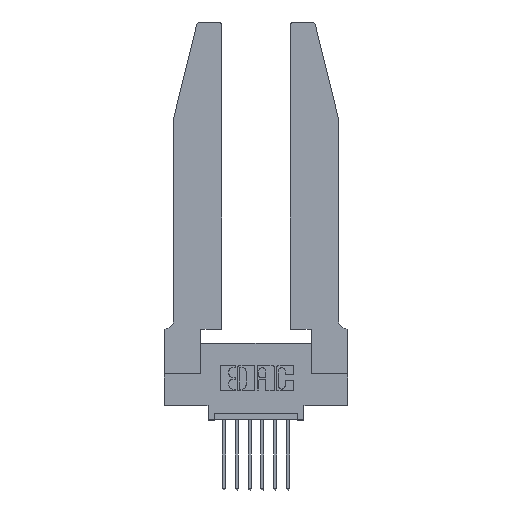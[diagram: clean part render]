
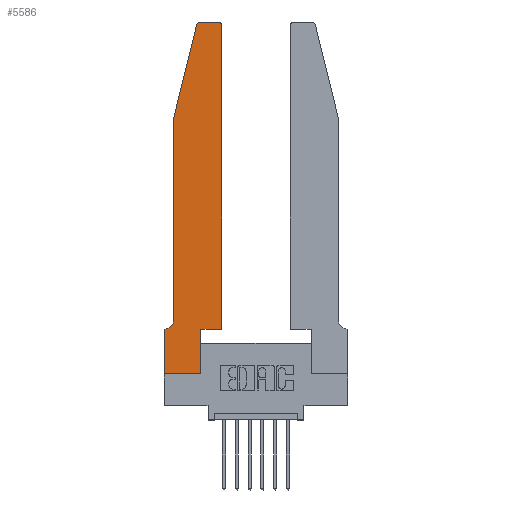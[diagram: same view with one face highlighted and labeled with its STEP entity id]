
A CAD part, top view. The second image highlights one B-rep face of the part: STEP entity #5586.
In plain terms, the highlighted planar face has unit normal (0, 0, 1).
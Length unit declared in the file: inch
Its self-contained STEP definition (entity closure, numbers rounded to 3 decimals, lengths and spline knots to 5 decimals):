
#193 = CARTESIAN_POINT ( 'NONE',  ( 0.4505, 2.72, 0.37 ) ) ;
#317 = EDGE_CURVE ( 'NONE', #8953, #6873, #13744, .T. ) ;
#585 = DIRECTION ( 'NONE',  ( 0., 1., 0. ) ) ;
#881 = CARTESIAN_POINT ( 'NONE',  ( 0.0055, 0.35, 0.37 ) ) ;
#1132 = DIRECTION ( 'NONE',  ( 1., 0., 0. ) ) ;
#1405 = VERTEX_POINT ( 'NONE', #6700 ) ;
#1771 = EDGE_CURVE ( 'NONE', #5127, #13614, #2562, .T. ) ;
#1801 = VECTOR ( 'NONE', #3980, 39.37008 ) ;
#2337 = DIRECTION ( 'NONE',  ( -1., 0., 0. ) ) ;
#2392 = CARTESIAN_POINT ( 'NONE',  ( 0.0755, 0.35, 0.37 ) ) ;
#2511 = LINE ( 'NONE', #11585, #11950 ) ;
#2553 = DIRECTION ( 'NONE',  ( 0., 1., 0. ) ) ;
#2562 = LINE ( 'NONE', #3612, #6663 ) ;
#2755 = VERTEX_POINT ( 'NONE', #8130 ) ;
#2925 = VECTOR ( 'NONE', #13827, 39.37008 ) ;
#3608 = EDGE_CURVE ( 'NONE', #11274, #7448, #2511, .T. ) ;
#3612 = CARTESIAN_POINT ( 'NONE',  ( 0., 0., 0.37 ) ) ;
#3656 = CARTESIAN_POINT ( 'NONE',  ( 0.0755, 2., 0.37 ) ) ;
#3699 = VECTOR ( 'NONE', #13794, 39.37008 ) ;
#3912 = CARTESIAN_POINT ( 'NONE',  ( 0., 0.35, 0.37 ) ) ;
#3980 = DIRECTION ( 'NONE',  ( 1., 0., 0. ) ) ;
#4232 = AXIS2_PLACEMENT_3D ( 'NONE', #11447, #13595, #7993 ) ;
#4263 = DIRECTION ( 'NONE',  ( 0., 0., 1. ) ) ;
#4504 = ORIENTED_EDGE ( 'NONE', *, *, #13105, .T. ) ;
#4543 = EDGE_CURVE ( 'NONE', #13614, #11274, #11065, .T. ) ;
#4575 = EDGE_CURVE ( 'NONE', #5020, #2755, #6593, .T. ) ;
#4583 = VECTOR ( 'NONE', #9772, 39.37008 ) ;
#4726 = EDGE_CURVE ( 'NONE', #6873, #5210, #8148, .T. ) ;
#4813 = LINE ( 'NONE', #9290, #2925 ) ;
#4885 = EDGE_CURVE ( 'NONE', #2755, #11107, #7281, .T. ) ;
#5020 = VERTEX_POINT ( 'NONE', #12413 ) ;
#5127 = VERTEX_POINT ( 'NONE', #3912 ) ;
#5210 = VERTEX_POINT ( 'NONE', #13983 ) ;
#5295 = VECTOR ( 'NONE', #2553, 39.37008 ) ;
#5488 = AXIS2_PLACEMENT_3D ( 'NONE', #7690, #4263, #1132 ) ;
#5586 = ADVANCED_FACE ( 'NONE', ( #7943 ), #8099, .T. ) ;
#5783 = CARTESIAN_POINT ( 'NONE',  ( 0., 0., 0.37 ) ) ;
#5892 = ORIENTED_EDGE ( 'NONE', *, *, #4575, .T. ) ;
#5915 = VERTEX_POINT ( 'NONE', #9154 ) ;
#6064 = CARTESIAN_POINT ( 'NONE',  ( 0.2865, 0.35, 0.37 ) ) ;
#6113 = DIRECTION ( 'NONE',  ( 0., 0., 1. ) ) ;
#6593 = LINE ( 'NONE', #8356, #3699 ) ;
#6663 = VECTOR ( 'NONE', #12492, 39.37008 ) ;
#6700 = CARTESIAN_POINT ( 'NONE',  ( 0.25487, 2.72718, 0.37 ) ) ;
#6873 = VERTEX_POINT ( 'NONE', #193 ) ;
#6919 = CARTESIAN_POINT ( 'NONE',  ( 0.4505, 0.35, 0.37 ) ) ;
#7006 = CARTESIAN_POINT ( 'NONE',  ( 0., 0., 0.37 ) ) ;
#7033 = EDGE_CURVE ( 'NONE', #7448, #8953, #4813, .T. ) ;
#7281 = CIRCLE ( 'NONE', #14024, 0.07 ) ;
#7448 = VERTEX_POINT ( 'NONE', #6064 ) ;
#7690 = CARTESIAN_POINT ( 'NONE',  ( 0.4205, 2.72, 0.37 ) ) ;
#7939 = DIRECTION ( 'NONE',  ( 0., 0., -1. ) ) ;
#7943 = FACE_OUTER_BOUND ( 'NONE', #8574, .T. ) ;
#7993 = DIRECTION ( 'NONE',  ( 1., 0., 0. ) ) ;
#8099 = PLANE ( 'NONE',  #4232 ) ;
#8130 = CARTESIAN_POINT ( 'NONE',  ( 0.0755, 0.42, 0.37 ) ) ;
#8148 = CIRCLE ( 'NONE', #5488, 0.03 ) ;
#8356 = CARTESIAN_POINT ( 'NONE',  ( 0.0755, 2., 0.37 ) ) ;
#8435 = ORIENTED_EDGE ( 'NONE', *, *, #4885, .T. ) ;
#8574 = EDGE_LOOP ( 'NONE', ( #4504, #12296, #8700, #5892, #8435, #14189, #14200, #13268, #10873, #9449, #9288, #9050 ) ) ;
#8700 = ORIENTED_EDGE ( 'NONE', *, *, #10492, .T. ) ;
#8719 = VECTOR ( 'NONE', #12751, 39.37008 ) ;
#8953 = VERTEX_POINT ( 'NONE', #13448 ) ;
#9050 = ORIENTED_EDGE ( 'NONE', *, *, #4726, .T. ) ;
#9154 = CARTESIAN_POINT ( 'NONE',  ( 0.284, 2.75, 0.37 ) ) ;
#9288 = ORIENTED_EDGE ( 'NONE', *, *, #317, .T. ) ;
#9290 = CARTESIAN_POINT ( 'NONE',  ( 0.4505, 0.35, 0.37 ) ) ;
#9449 = ORIENTED_EDGE ( 'NONE', *, *, #7033, .T. ) ;
#9772 = DIRECTION ( 'NONE',  ( -1., 0., 0. ) ) ;
#9961 = VECTOR ( 'NONE', #13559, 39.37008 ) ;
#9978 = CIRCLE ( 'NONE', #12562, 0.03 ) ;
#10241 = EDGE_CURVE ( 'NONE', #5915, #1405, #9978, .T. ) ;
#10492 = EDGE_CURVE ( 'NONE', #1405, #5020, #12743, .T. ) ;
#10873 = ORIENTED_EDGE ( 'NONE', *, *, #3608, .T. ) ;
#11065 = LINE ( 'NONE', #5783, #1801 ) ;
#11099 = LINE ( 'NONE', #2392, #4583 ) ;
#11107 = VERTEX_POINT ( 'NONE', #881 ) ;
#11274 = VERTEX_POINT ( 'NONE', #13874 ) ;
#11447 = CARTESIAN_POINT ( 'NONE',  ( 0., 0.35, 0.37 ) ) ;
#11585 = CARTESIAN_POINT ( 'NONE',  ( 0.2865, 0.35, 0.37 ) ) ;
#11768 = CARTESIAN_POINT ( 'NONE',  ( 0.2605, 2.75, 0.37 ) ) ;
#11950 = VECTOR ( 'NONE', #585, 39.37008 ) ;
#12260 = CARTESIAN_POINT ( 'NONE',  ( 0.0055, 0.42, 0.37 ) ) ;
#12296 = ORIENTED_EDGE ( 'NONE', *, *, #10241, .T. ) ;
#12413 = CARTESIAN_POINT ( 'NONE',  ( 0.0755, 2., 0.37 ) ) ;
#12492 = DIRECTION ( 'NONE',  ( 0., -1., 0. ) ) ;
#12562 = AXIS2_PLACEMENT_3D ( 'NONE', #12718, #6113, #13849 ) ;
#12718 = CARTESIAN_POINT ( 'NONE',  ( 0.284, 2.72, 0.37 ) ) ;
#12743 = LINE ( 'NONE', #3656, #9961 ) ;
#12751 = DIRECTION ( 'NONE',  ( -1., 0., 0. ) ) ;
#13004 = LINE ( 'NONE', #11768, #8719 ) ;
#13105 = EDGE_CURVE ( 'NONE', #5210, #5915, #13004, .T. ) ;
#13268 = ORIENTED_EDGE ( 'NONE', *, *, #4543, .T. ) ;
#13448 = CARTESIAN_POINT ( 'NONE',  ( 0.4505, 0.35, 0.37 ) ) ;
#13559 = DIRECTION ( 'NONE',  ( -0.239, -0.971, 0. ) ) ;
#13595 = DIRECTION ( 'NONE',  ( 0., 0., 1. ) ) ;
#13614 = VERTEX_POINT ( 'NONE', #7006 ) ;
#13744 = LINE ( 'NONE', #6919, #5295 ) ;
#13794 = DIRECTION ( 'NONE',  ( 0., -1., 0. ) ) ;
#13827 = DIRECTION ( 'NONE',  ( 1., 0., 0. ) ) ;
#13849 = DIRECTION ( 'NONE',  ( 1., 0., 0. ) ) ;
#13874 = CARTESIAN_POINT ( 'NONE',  ( 0.2865, 0., 0.37 ) ) ;
#13983 = CARTESIAN_POINT ( 'NONE',  ( 0.4205, 2.75, 0.37 ) ) ;
#14024 = AXIS2_PLACEMENT_3D ( 'NONE', #12260, #7939, #2337 ) ;
#14067 = EDGE_CURVE ( 'NONE', #11107, #5127, #11099, .T. ) ;
#14189 = ORIENTED_EDGE ( 'NONE', *, *, #14067, .T. ) ;
#14200 = ORIENTED_EDGE ( 'NONE', *, *, #1771, .T. ) ;
